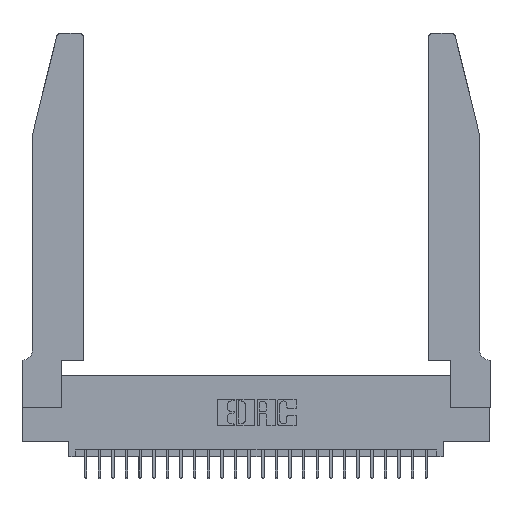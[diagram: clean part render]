
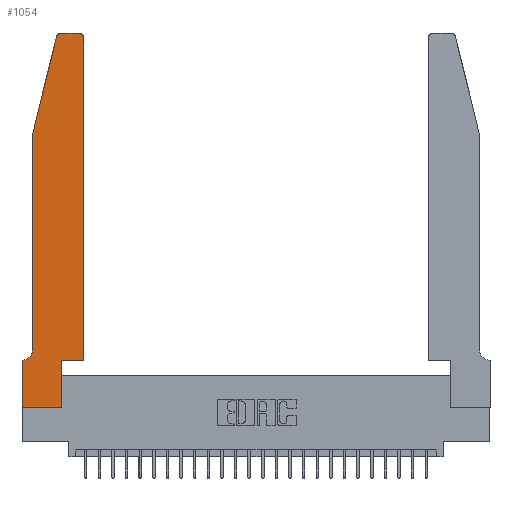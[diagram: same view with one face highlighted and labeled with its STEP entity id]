
A CAD part, top view. The second image highlights one B-rep face of the part: STEP entity #1054.
In plain terms, the highlighted planar face has unit normal (0, 0, 1).
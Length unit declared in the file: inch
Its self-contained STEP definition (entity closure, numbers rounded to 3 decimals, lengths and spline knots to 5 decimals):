
#34 = LINE ( 'NONE', #7121, #22129 ) ;
#821 = CARTESIAN_POINT ( 'NONE',  ( 0.4205, 2.72, 0.37 ) ) ;
#971 = VECTOR ( 'NONE', #15324, 39.37008 ) ;
#976 = ORIENTED_EDGE ( 'NONE', *, *, #7787, .T. ) ;
#1004 = CARTESIAN_POINT ( 'NONE',  ( 0.0755, 2., 0.37 ) ) ;
#1054 = ADVANCED_FACE ( 'NONE', ( #9524 ), #5268, .T. ) ;
#1251 = LINE ( 'NONE', #3412, #17775 ) ;
#1643 = AXIS2_PLACEMENT_3D ( 'NONE', #15924, #3000, #17975 ) ;
#1687 = AXIS2_PLACEMENT_3D ( 'NONE', #16056, #3149, #18106 ) ;
#2027 = VECTOR ( 'NONE', #6763, 39.37008 ) ;
#2326 = VERTEX_POINT ( 'NONE', #1004 ) ;
#2555 = LINE ( 'NONE', #9584, #13490 ) ;
#2931 = DIRECTION ( 'NONE',  ( 1., 0., 0. ) ) ;
#2944 = CIRCLE ( 'NONE', #21775, 0.03 ) ;
#3000 = DIRECTION ( 'NONE',  ( 0., 0., 1. ) ) ;
#3136 = DIRECTION ( 'NONE',  ( 1., 0., 0. ) ) ;
#3149 = DIRECTION ( 'NONE',  ( 0., 0., -1. ) ) ;
#3412 = CARTESIAN_POINT ( 'NONE',  ( 0.2865, 0.35, 0.37 ) ) ;
#4682 = AXIS2_PLACEMENT_3D ( 'NONE', #13915, #27465, #2931 ) ;
#4837 = LINE ( 'NONE', #17245, #25803 ) ;
#5168 = VERTEX_POINT ( 'NONE', #16456 ) ;
#5268 = PLANE ( 'NONE',  #4682 ) ;
#5602 = VECTOR ( 'NONE', #13836, 39.37008 ) ;
#6763 = DIRECTION ( 'NONE',  ( 1., 0., 0. ) ) ;
#6987 = CARTESIAN_POINT ( 'NONE',  ( 0., 0.35, 0.37 ) ) ;
#7121 = CARTESIAN_POINT ( 'NONE',  ( 0., 0., 0.37 ) ) ;
#7502 = DIRECTION ( 'NONE',  ( 0., 1., 0. ) ) ;
#7517 = CARTESIAN_POINT ( 'NONE',  ( 0.0755, 2., 0.37 ) ) ;
#7645 = ORIENTED_EDGE ( 'NONE', *, *, #8806, .T. ) ;
#7787 = EDGE_CURVE ( 'NONE', #9935, #2326, #16913, .T. ) ;
#7794 = VERTEX_POINT ( 'NONE', #9696 ) ;
#8025 = LINE ( 'NONE', #27506, #2027 ) ;
#8806 = EDGE_CURVE ( 'NONE', #2326, #13643, #18182, .T. ) ;
#8994 = CARTESIAN_POINT ( 'NONE',  ( 0.0755, 2., 0.37 ) ) ;
#9524 = FACE_OUTER_BOUND ( 'NONE', #17342, .T. ) ;
#9584 = CARTESIAN_POINT ( 'NONE',  ( 0.4505, 0.35, 0.37 ) ) ;
#9696 = CARTESIAN_POINT ( 'NONE',  ( 0.2865, 0.35, 0.37 ) ) ;
#9817 = EDGE_CURVE ( 'NONE', #16562, #12972, #4837, .T. ) ;
#9935 = VERTEX_POINT ( 'NONE', #25824 ) ;
#10920 = ORIENTED_EDGE ( 'NONE', *, *, #13935, .T. ) ;
#11358 = CARTESIAN_POINT ( 'NONE',  ( 0.4505, 0.35, 0.37 ) ) ;
#12712 = EDGE_CURVE ( 'NONE', #5168, #16562, #2944, .T. ) ;
#12972 = VERTEX_POINT ( 'NONE', #24945 ) ;
#13348 = EDGE_CURVE ( 'NONE', #12972, #9935, #25654, .T. ) ;
#13490 = VECTOR ( 'NONE', #7502, 39.37008 ) ;
#13555 = ORIENTED_EDGE ( 'NONE', *, *, #21925, .T. ) ;
#13643 = VERTEX_POINT ( 'NONE', #27021 ) ;
#13689 = ORIENTED_EDGE ( 'NONE', *, *, #20394, .T. ) ;
#13796 = DIRECTION ( 'NONE',  ( 0., -1., 0. ) ) ;
#13836 = DIRECTION ( 'NONE',  ( -0.239, -0.971, 0. ) ) ;
#13915 = CARTESIAN_POINT ( 'NONE',  ( 0., 0.35, 0.37 ) ) ;
#13935 = EDGE_CURVE ( 'NONE', #22790, #20271, #23685, .T. ) ;
#14332 = LINE ( 'NONE', #26054, #19738 ) ;
#14764 = EDGE_CURVE ( 'NONE', #7794, #17598, #8025, .T. ) ;
#15324 = DIRECTION ( 'NONE',  ( 0., -1., 0. ) ) ;
#15795 = EDGE_CURVE ( 'NONE', #13643, #22790, #27392, .T. ) ;
#15924 = CARTESIAN_POINT ( 'NONE',  ( 0.284, 2.72, 0.37 ) ) ;
#15944 = ORIENTED_EDGE ( 'NONE', *, *, #14764, .T. ) ;
#15968 = ORIENTED_EDGE ( 'NONE', *, *, #17993, .T. ) ;
#16049 = DIRECTION ( 'NONE',  ( 0., 0., 1. ) ) ;
#16056 = CARTESIAN_POINT ( 'NONE',  ( 0.0055, 0.42, 0.37 ) ) ;
#16456 = CARTESIAN_POINT ( 'NONE',  ( 0.4505, 2.72, 0.37 ) ) ;
#16562 = VERTEX_POINT ( 'NONE', #26482 ) ;
#16913 = LINE ( 'NONE', #7517, #5602 ) ;
#17245 = CARTESIAN_POINT ( 'NONE',  ( 0.2605, 2.75, 0.37 ) ) ;
#17332 = DIRECTION ( 'NONE',  ( -1., 0., 0. ) ) ;
#17342 = EDGE_LOOP ( 'NONE', ( #22015, #18283, #976, #7645, #21567, #10920, #13689, #15968, #13555, #15944, #21528, #21353 ) ) ;
#17598 = VERTEX_POINT ( 'NONE', #11358 ) ;
#17775 = VECTOR ( 'NONE', #26397, 39.37008 ) ;
#17975 = DIRECTION ( 'NONE',  ( 1., 0., 0. ) ) ;
#17993 = EDGE_CURVE ( 'NONE', #25420, #21264, #34, .T. ) ;
#18106 = DIRECTION ( 'NONE',  ( -1., 0., 0. ) ) ;
#18118 = EDGE_CURVE ( 'NONE', #17598, #5168, #2555, .T. ) ;
#18182 = LINE ( 'NONE', #8994, #971 ) ;
#18283 = ORIENTED_EDGE ( 'NONE', *, *, #13348, .T. ) ;
#19623 = DIRECTION ( 'NONE',  ( 1., 0., 0. ) ) ;
#19738 = VECTOR ( 'NONE', #13796, 39.37008 ) ;
#20271 = VERTEX_POINT ( 'NONE', #6987 ) ;
#20394 = EDGE_CURVE ( 'NONE', #20271, #25420, #14332, .T. ) ;
#21264 = VERTEX_POINT ( 'NONE', #26608 ) ;
#21353 = ORIENTED_EDGE ( 'NONE', *, *, #12712, .T. ) ;
#21528 = ORIENTED_EDGE ( 'NONE', *, *, #18118, .T. ) ;
#21567 = ORIENTED_EDGE ( 'NONE', *, *, #15795, .T. ) ;
#21775 = AXIS2_PLACEMENT_3D ( 'NONE', #821, #16049, #3136 ) ;
#21865 = CARTESIAN_POINT ( 'NONE',  ( 0.0755, 0.35, 0.37 ) ) ;
#21925 = EDGE_CURVE ( 'NONE', #21264, #7794, #1251, .T. ) ;
#22015 = ORIENTED_EDGE ( 'NONE', *, *, #9817, .T. ) ;
#22129 = VECTOR ( 'NONE', #19623, 39.37008 ) ;
#22790 = VERTEX_POINT ( 'NONE', #23375 ) ;
#23046 = VECTOR ( 'NONE', #23921, 39.37008 ) ;
#23375 = CARTESIAN_POINT ( 'NONE',  ( 0.0055, 0.35, 0.37 ) ) ;
#23685 = LINE ( 'NONE', #21865, #23046 ) ;
#23921 = DIRECTION ( 'NONE',  ( -1., 0., 0. ) ) ;
#24945 = CARTESIAN_POINT ( 'NONE',  ( 0.284, 2.75, 0.37 ) ) ;
#25420 = VERTEX_POINT ( 'NONE', #25904 ) ;
#25654 = CIRCLE ( 'NONE', #1643, 0.03 ) ;
#25803 = VECTOR ( 'NONE', #17332, 39.37008 ) ;
#25824 = CARTESIAN_POINT ( 'NONE',  ( 0.25487, 2.72718, 0.37 ) ) ;
#25904 = CARTESIAN_POINT ( 'NONE',  ( 0., 0., 0.37 ) ) ;
#26054 = CARTESIAN_POINT ( 'NONE',  ( 0., 0., 0.37 ) ) ;
#26397 = DIRECTION ( 'NONE',  ( 0., 1., 0. ) ) ;
#26482 = CARTESIAN_POINT ( 'NONE',  ( 0.4205, 2.75, 0.37 ) ) ;
#26608 = CARTESIAN_POINT ( 'NONE',  ( 0.2865, 0., 0.37 ) ) ;
#27021 = CARTESIAN_POINT ( 'NONE',  ( 0.0755, 0.42, 0.37 ) ) ;
#27392 = CIRCLE ( 'NONE', #1687, 0.07 ) ;
#27465 = DIRECTION ( 'NONE',  ( 0., 0., 1. ) ) ;
#27506 = CARTESIAN_POINT ( 'NONE',  ( 0.4505, 0.35, 0.37 ) ) ;
